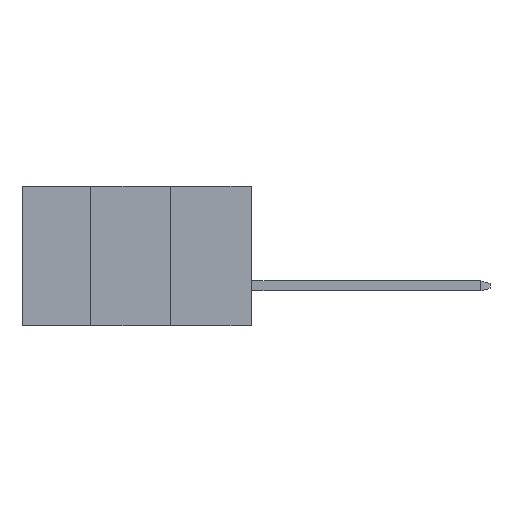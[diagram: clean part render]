
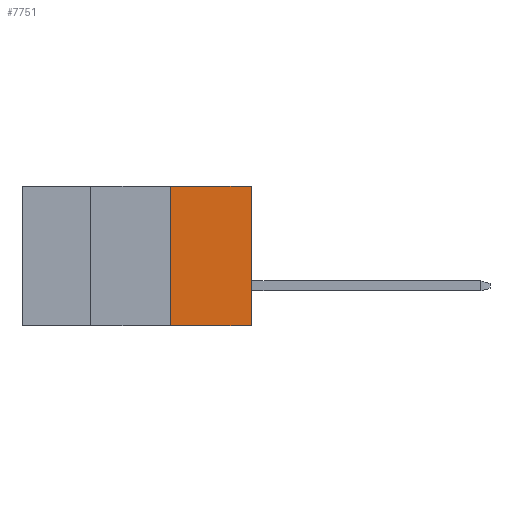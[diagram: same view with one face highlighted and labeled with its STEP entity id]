
A CAD part, left-side view. The second image highlights one B-rep face of the part: STEP entity #7751.
In plain terms, the highlighted planar face has unit normal (-1, 0, 0).
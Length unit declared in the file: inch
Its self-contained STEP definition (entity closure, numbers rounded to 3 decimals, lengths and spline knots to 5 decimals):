
#293 = VECTOR ( 'NONE', #1527, 39.37008 ) ;
#345 = EDGE_LOOP ( 'NONE', ( #4115, #6757, #2720, #6556 ) ) ;
#767 = VERTEX_POINT ( 'NONE', #8110 ) ;
#956 = VERTEX_POINT ( 'NONE', #6488 ) ;
#1443 = VECTOR ( 'NONE', #6010, 39.37008 ) ;
#1495 = DIRECTION ( 'NONE',  ( 1., 0., 0. ) ) ;
#1527 = DIRECTION ( 'NONE',  ( 0., 0., 1. ) ) ;
#1583 = VERTEX_POINT ( 'NONE', #3091 ) ;
#2151 = EDGE_CURVE ( 'NONE', #767, #1583, #2527, .T. ) ;
#2152 = EDGE_CURVE ( 'NONE', #956, #5517, #4608, .T. ) ;
#2166 = FACE_OUTER_BOUND ( 'NONE', #345, .T. ) ;
#2189 = CARTESIAN_POINT ( 'NONE',  ( 0.4265, 0., -0.437 ) ) ;
#2527 = LINE ( 'NONE', #5293, #4453 ) ;
#2720 = ORIENTED_EDGE ( 'NONE', *, *, #7488, .F. ) ;
#2970 = CARTESIAN_POINT ( 'NONE',  ( 0.4265, 0., -0.437 ) ) ;
#3091 = CARTESIAN_POINT ( 'NONE',  ( 0.4265, 0., 0. ) ) ;
#3563 = PLANE ( 'NONE',  #8656 ) ;
#4115 = ORIENTED_EDGE ( 'NONE', *, *, #4251, .T. ) ;
#4198 = DIRECTION ( 'NONE',  ( 0., 0., 1. ) ) ;
#4242 = DIRECTION ( 'NONE',  ( 0., 0., -1. ) ) ;
#4251 = EDGE_CURVE ( 'NONE', #5517, #1583, #7106, .T. ) ;
#4281 = CARTESIAN_POINT ( 'NONE',  ( 0.4265, 0.254, -0.437 ) ) ;
#4453 = VECTOR ( 'NONE', #5155, 39.37008 ) ;
#4608 = LINE ( 'NONE', #7252, #1443 ) ;
#4701 = CARTESIAN_POINT ( 'NONE',  ( 0.4265, 0.254, -0.437 ) ) ;
#4962 = VECTOR ( 'NONE', #4198, 39.37008 ) ;
#5155 = DIRECTION ( 'NONE',  ( 0., -1., 0. ) ) ;
#5293 = CARTESIAN_POINT ( 'NONE',  ( 0.4265, 0.254, 0. ) ) ;
#5517 = VERTEX_POINT ( 'NONE', #2189 ) ;
#6010 = DIRECTION ( 'NONE',  ( 0., -1., 0. ) ) ;
#6488 = CARTESIAN_POINT ( 'NONE',  ( 0.4265, 0.254, -0.437 ) ) ;
#6556 = ORIENTED_EDGE ( 'NONE', *, *, #2152, .T. ) ;
#6757 = ORIENTED_EDGE ( 'NONE', *, *, #2151, .F. ) ;
#7106 = LINE ( 'NONE', #2970, #293 ) ;
#7252 = CARTESIAN_POINT ( 'NONE',  ( 0.4265, 0.254, -0.437 ) ) ;
#7475 = LINE ( 'NONE', #4701, #4962 ) ;
#7488 = EDGE_CURVE ( 'NONE', #956, #767, #7475, .T. ) ;
#7751 = ADVANCED_FACE ( 'NONE', ( #2166 ), #3563, .F. ) ;
#8110 = CARTESIAN_POINT ( 'NONE',  ( 0.4265, 0.254, 0. ) ) ;
#8656 = AXIS2_PLACEMENT_3D ( 'NONE', #4281, #1495, #4242 ) ;
